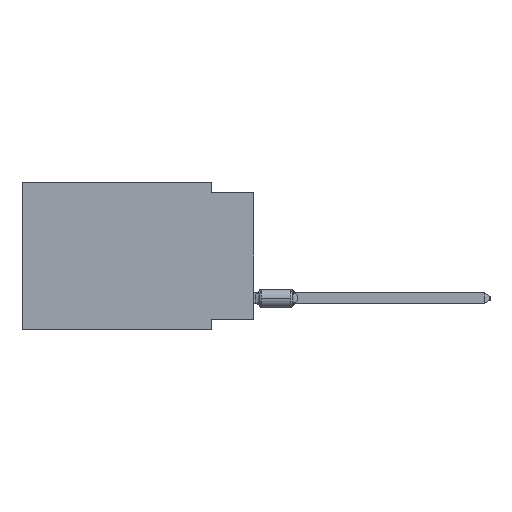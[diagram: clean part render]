
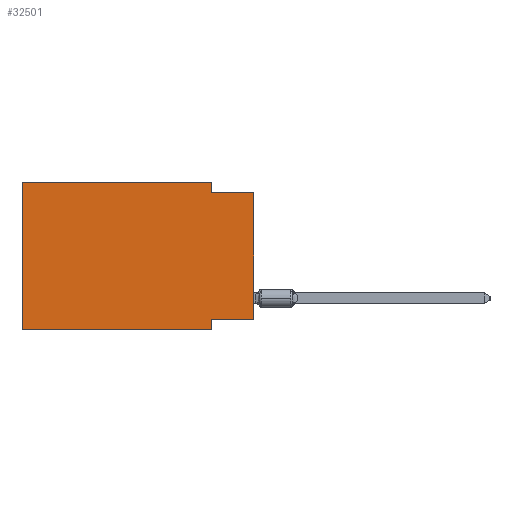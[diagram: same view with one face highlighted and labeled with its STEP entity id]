
A CAD part, left-side view. The second image highlights one B-rep face of the part: STEP entity #32501.
In plain terms, the highlighted planar face has unit normal (-1, 0, 0).
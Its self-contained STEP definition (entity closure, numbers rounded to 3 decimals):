
#611 = CARTESIAN_POINT ( 'NONE',  ( 0., 13.97, 0. ) ) ;
#1157 = CARTESIAN_POINT ( 'NONE',  ( 0., 2.54, 0. ) ) ;
#1431 = VECTOR ( 'NONE', #36084, 1000. ) ;
#1710 = CARTESIAN_POINT ( 'NONE',  ( 0., 2.54, -8.255 ) ) ;
#1880 = CARTESIAN_POINT ( 'NONE',  ( 0., 0., -0.635 ) ) ;
#1955 = CARTESIAN_POINT ( 'NONE',  ( 0., 13.97, -8.89 ) ) ;
#5723 = LINE ( 'NONE', #18885, #35029 ) ;
#5813 = EDGE_CURVE ( 'NONE', #33501, #24500, #19319, .T. ) ;
#5889 = VERTEX_POINT ( 'NONE', #1955 ) ;
#7002 = DIRECTION ( 'NONE',  ( 0., 0., -1. ) ) ;
#7416 = EDGE_CURVE ( 'NONE', #5889, #31860, #5723, .T. ) ;
#8732 = FACE_OUTER_BOUND ( 'NONE', #30034, .T. ) ;
#9521 = VECTOR ( 'NONE', #34345, 1000. ) ;
#9601 = CARTESIAN_POINT ( 'NONE',  ( 0., 13.97, -8.89 ) ) ;
#9999 = VECTOR ( 'NONE', #7002, 1000. ) ;
#10148 = VECTOR ( 'NONE', #21601, 1000. ) ;
#10978 = ORIENTED_EDGE ( 'NONE', *, *, #36501, .F. ) ;
#10991 = CARTESIAN_POINT ( 'NONE',  ( 0., 2.54, -8.89 ) ) ;
#11014 = EDGE_CURVE ( 'NONE', #18421, #16269, #16093, .T. ) ;
#11652 = LINE ( 'NONE', #20350, #18459 ) ;
#11706 = VECTOR ( 'NONE', #26764, 1000. ) ;
#11908 = ORIENTED_EDGE ( 'NONE', *, *, #23258, .F. ) ;
#15142 = VERTEX_POINT ( 'NONE', #22260 ) ;
#16081 = VECTOR ( 'NONE', #22123, 1000. ) ;
#16093 = LINE ( 'NONE', #30513, #9999 ) ;
#16178 = CARTESIAN_POINT ( 'NONE',  ( 0., 0., -8.255 ) ) ;
#16269 = VERTEX_POINT ( 'NONE', #19229 ) ;
#17621 = DIRECTION ( 'NONE',  ( 0., 0., -1. ) ) ;
#17771 = ORIENTED_EDGE ( 'NONE', *, *, #19328, .F. ) ;
#18421 = VERTEX_POINT ( 'NONE', #1157 ) ;
#18459 = VECTOR ( 'NONE', #23712, 1000. ) ;
#18885 = CARTESIAN_POINT ( 'NONE',  ( 0., 13.97, 0. ) ) ;
#19229 = CARTESIAN_POINT ( 'NONE',  ( 0., 2.54, -0.635 ) ) ;
#19319 = LINE ( 'NONE', #16178, #9521 ) ;
#19328 = EDGE_CURVE ( 'NONE', #24500, #15142, #38037, .T. ) ;
#20350 = CARTESIAN_POINT ( 'NONE',  ( 0., 0., 0. ) ) ;
#21543 = ORIENTED_EDGE ( 'NONE', *, *, #25063, .T. ) ;
#21601 = DIRECTION ( 'NONE',  ( 0., -1., 0. ) ) ;
#21849 = CARTESIAN_POINT ( 'NONE',  ( 0., 13.97, 0. ) ) ;
#22123 = DIRECTION ( 'NONE',  ( 0., -1., 0. ) ) ;
#22260 = CARTESIAN_POINT ( 'NONE',  ( 0., 2.54, -8.89 ) ) ;
#23258 = EDGE_CURVE ( 'NONE', #16269, #30617, #24957, .T. ) ;
#23555 = DIRECTION ( 'NONE',  ( 1., 0., 0. ) ) ;
#23712 = DIRECTION ( 'NONE',  ( 0., 0., 1. ) ) ;
#23845 = CARTESIAN_POINT ( 'NONE',  ( 0., 0., -0.635 ) ) ;
#24449 = EDGE_CURVE ( 'NONE', #5889, #15142, #36662, .T. ) ;
#24500 = VERTEX_POINT ( 'NONE', #1710 ) ;
#24957 = LINE ( 'NONE', #23845, #10148 ) ;
#25063 = EDGE_CURVE ( 'NONE', #33501, #30617, #11652, .T. ) ;
#25422 = ORIENTED_EDGE ( 'NONE', *, *, #5813, .F. ) ;
#26764 = DIRECTION ( 'NONE',  ( 0., 0., -1. ) ) ;
#26895 = CARTESIAN_POINT ( 'NONE',  ( 0., 13.97, 0. ) ) ;
#28247 = LINE ( 'NONE', #611, #16081 ) ;
#30034 = EDGE_LOOP ( 'NONE', ( #21543, #11908, #30668, #10978, #35887, #34192, #17771, #25422 ) ) ;
#30498 = CARTESIAN_POINT ( 'NONE',  ( 0., 0., -8.255 ) ) ;
#30513 = CARTESIAN_POINT ( 'NONE',  ( 0., 2.54, 0. ) ) ;
#30617 = VERTEX_POINT ( 'NONE', #1880 ) ;
#30668 = ORIENTED_EDGE ( 'NONE', *, *, #11014, .F. ) ;
#31105 = AXIS2_PLACEMENT_3D ( 'NONE', #26895, #23555, #17621 ) ;
#31860 = VERTEX_POINT ( 'NONE', #21849 ) ;
#32501 = ADVANCED_FACE ( 'NONE', ( #8732 ), #35411, .F. ) ;
#33501 = VERTEX_POINT ( 'NONE', #30498 ) ;
#34192 = ORIENTED_EDGE ( 'NONE', *, *, #24449, .T. ) ;
#34345 = DIRECTION ( 'NONE',  ( 0., 1., 0. ) ) ;
#35029 = VECTOR ( 'NONE', #35946, 1000. ) ;
#35411 = PLANE ( 'NONE',  #31105 ) ;
#35887 = ORIENTED_EDGE ( 'NONE', *, *, #7416, .F. ) ;
#35946 = DIRECTION ( 'NONE',  ( 0., 0., 1. ) ) ;
#36084 = DIRECTION ( 'NONE',  ( 0., -1., 0. ) ) ;
#36501 = EDGE_CURVE ( 'NONE', #31860, #18421, #28247, .T. ) ;
#36662 = LINE ( 'NONE', #9601, #1431 ) ;
#38037 = LINE ( 'NONE', #10991, #11706 ) ;
